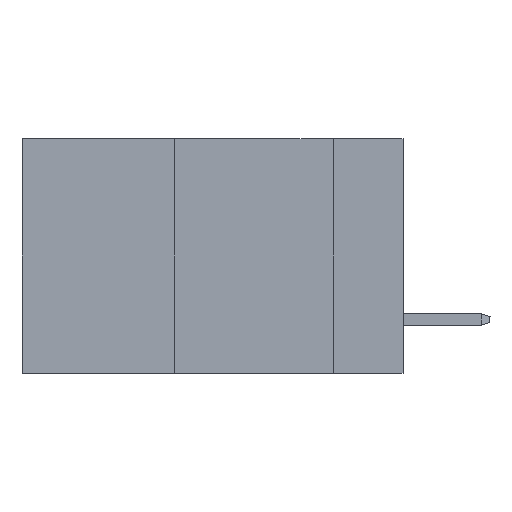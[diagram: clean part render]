
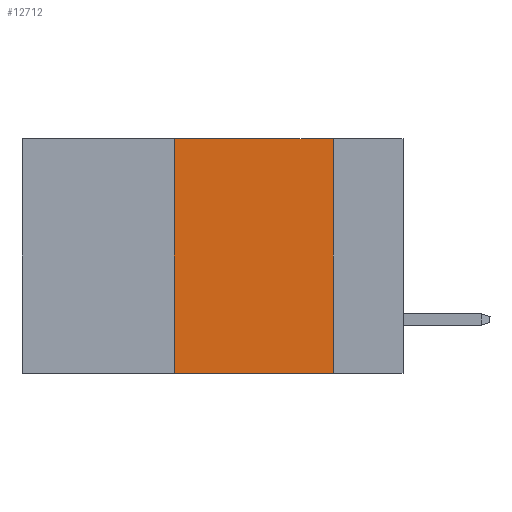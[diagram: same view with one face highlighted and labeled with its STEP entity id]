
A CAD part, left-side view. The second image highlights one B-rep face of the part: STEP entity #12712.
In plain terms, the highlighted planar face has unit normal (-1, 0, 0).
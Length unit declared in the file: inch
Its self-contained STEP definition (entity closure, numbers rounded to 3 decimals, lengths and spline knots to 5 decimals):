
#321 = VECTOR ( 'NONE', #2992, 39.37008 ) ;
#1087 = EDGE_LOOP ( 'NONE', ( #16705, #5357, #2015, #12488 ) ) ;
#1452 = CARTESIAN_POINT ( 'NONE',  ( 0., 0.6, 0. ) ) ;
#1768 = EDGE_CURVE ( 'NONE', #2859, #10205, #8996, .T. ) ;
#2015 = ORIENTED_EDGE ( 'NONE', *, *, #12000, .F. ) ;
#2199 = DIRECTION ( 'NONE',  ( 0., 0., 1. ) ) ;
#2273 = DIRECTION ( 'NONE',  ( 0., -1., 0. ) ) ;
#2612 = VERTEX_POINT ( 'NONE', #11309 ) ;
#2859 = VERTEX_POINT ( 'NONE', #9199 ) ;
#2875 = CARTESIAN_POINT ( 'NONE',  ( 0., 0.6, 0. ) ) ;
#2992 = DIRECTION ( 'NONE',  ( 0., 0., -1. ) ) ;
#5051 = CARTESIAN_POINT ( 'NONE',  ( 0., 0.11, 0. ) ) ;
#5357 = ORIENTED_EDGE ( 'NONE', *, *, #15728, .F. ) ;
#6689 = LINE ( 'NONE', #5051, #321 ) ;
#6864 = VECTOR ( 'NONE', #11003, 39.37008 ) ;
#7383 = CARTESIAN_POINT ( 'NONE',  ( 0., 0.6, -0.37 ) ) ;
#7470 = PLANE ( 'NONE',  #10549 ) ;
#8996 = LINE ( 'NONE', #7383, #10491 ) ;
#8997 = CARTESIAN_POINT ( 'NONE',  ( 0., 0.36, 0. ) ) ;
#9115 = VECTOR ( 'NONE', #2199, 39.37008 ) ;
#9199 = CARTESIAN_POINT ( 'NONE',  ( 0., 0.36, -0.37 ) ) ;
#9682 = DIRECTION ( 'NONE',  ( 0., 0., -1. ) ) ;
#10205 = VERTEX_POINT ( 'NONE', #19156 ) ;
#10491 = VECTOR ( 'NONE', #2273, 39.37008 ) ;
#10549 = AXIS2_PLACEMENT_3D ( 'NONE', #1452, #10805, #9682 ) ;
#10805 = DIRECTION ( 'NONE',  ( 1., 0., 0. ) ) ;
#11003 = DIRECTION ( 'NONE',  ( 0., -1., 0. ) ) ;
#11309 = CARTESIAN_POINT ( 'NONE',  ( 0., 0.11, 0. ) ) ;
#12000 = EDGE_CURVE ( 'NONE', #2859, #19194, #15271, .T. ) ;
#12488 = ORIENTED_EDGE ( 'NONE', *, *, #1768, .T. ) ;
#12712 = ADVANCED_FACE ( 'NONE', ( #12925 ), #7470, .F. ) ;
#12925 = FACE_OUTER_BOUND ( 'NONE', #1087, .T. ) ;
#14338 = LINE ( 'NONE', #2875, #6864 ) ;
#15271 = LINE ( 'NONE', #16984, #9115 ) ;
#15728 = EDGE_CURVE ( 'NONE', #19194, #2612, #14338, .T. ) ;
#16705 = ORIENTED_EDGE ( 'NONE', *, *, #20979, .F. ) ;
#16984 = CARTESIAN_POINT ( 'NONE',  ( 0., 0.36, 0. ) ) ;
#19156 = CARTESIAN_POINT ( 'NONE',  ( 0., 0.11, -0.37 ) ) ;
#19194 = VERTEX_POINT ( 'NONE', #8997 ) ;
#20979 = EDGE_CURVE ( 'NONE', #2612, #10205, #6689, .T. ) ;
